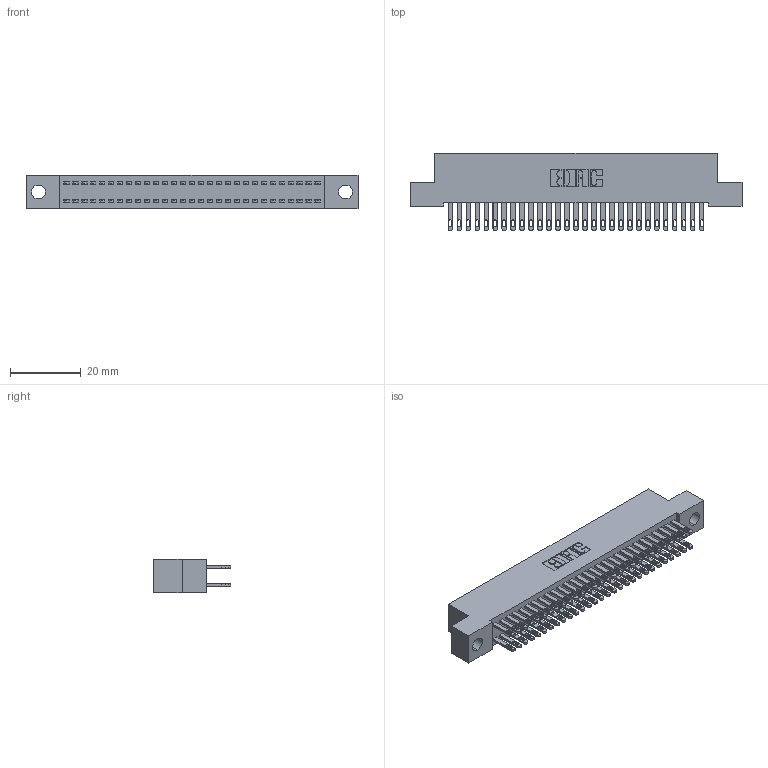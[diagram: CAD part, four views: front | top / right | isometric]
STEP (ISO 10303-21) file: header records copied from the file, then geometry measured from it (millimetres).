
FILE_DESCRIPTION (( 'STEP AP203' ), '1' );
FILE_NAME ('892-058-500-204.STEP', '2020-09-21T19:03:25', ( '' ), ( '' ), 'SwSTEP 2.0', 'SolidWorks 2020', '' );
FILE_SCHEMA (( 'CONFIG_CONTROL_DESIGN' ));
Length unit declared in the file: inch
Products named in the file (3): 892-058-500-204; 345-292-001_345-293-100; 842 Part_.156 TH
Assembly tree (59 placements, depth 2):
  892-058-500-204
    842 Part_.156 TH
    345-292-001_345-293-100  x58
Bounding box: 93.98 x 21.85 x 9.4 mm (x, y, z)
Volume: 8472.8 mm3; surface area: 13850.7 mm2
Topology: 59 solids, 59 shells, 2894 faces, 8825 edges, 5882 vertices
Faces by surface type: plane 1806, cylinder 1088
Entity records: 20139 total; most frequent: CARTESIAN_POINT 3350, ORIENTED_EDGE 3286, DIRECTION 2887, EDGE_CURVE 1643, LINE 1511, VECTOR 1511, VERTEX_POINT 1094, AXIS2_PLACEMENT_3D 688
